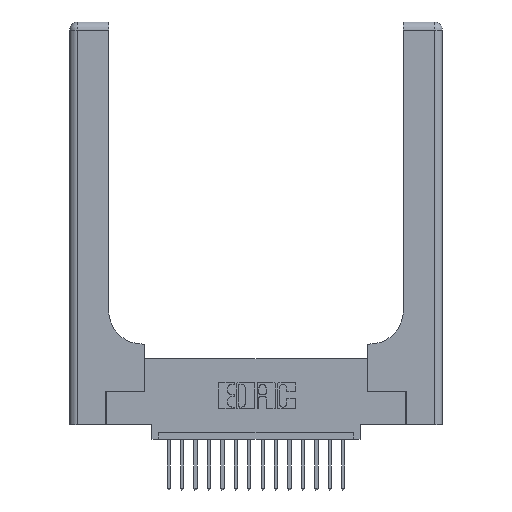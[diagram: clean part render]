
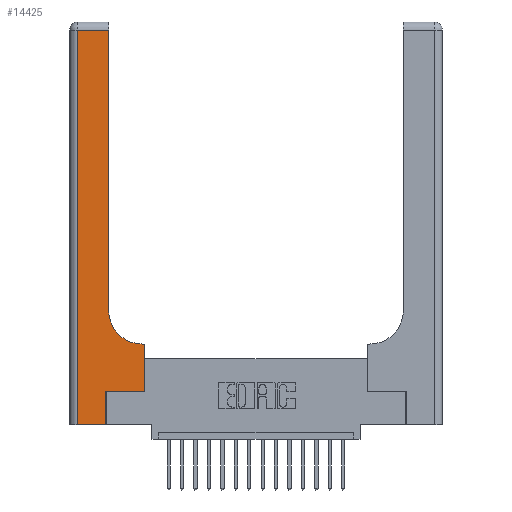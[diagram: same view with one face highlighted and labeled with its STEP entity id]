
A CAD part, top view. The second image highlights one B-rep face of the part: STEP entity #14425.
In plain terms, the highlighted planar face has unit normal (0, 0, 1).
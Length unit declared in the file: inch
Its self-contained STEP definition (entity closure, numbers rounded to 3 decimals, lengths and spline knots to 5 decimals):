
#74 = ORIENTED_EDGE ( 'NONE', *, *, #12690, .T. ) ;
#173 = CARTESIAN_POINT ( 'NONE',  ( 0.269, 0., 0.37 ) ) ;
#455 = CARTESIAN_POINT ( 'NONE',  ( 0.269, 0.25, 0.37 ) ) ;
#500 = EDGE_CURVE ( 'NONE', #16780, #14288, #3269, .T. ) ;
#541 = CARTESIAN_POINT ( 'NONE',  ( 0.5585, 0.25, 0.37 ) ) ;
#1495 = CARTESIAN_POINT ( 'NONE',  ( 0.5585, 0.25, 0.37 ) ) ;
#1512 = CARTESIAN_POINT ( 'NONE',  ( 0.269, 0., 0.37 ) ) ;
#1995 = DIRECTION ( 'NONE',  ( 1., 0., 0. ) ) ;
#2474 = LINE ( 'NONE', #9490, #4388 ) ;
#2658 = EDGE_CURVE ( 'NONE', #5302, #15532, #2474, .T. ) ;
#3269 = LINE ( 'NONE', #1495, #10329 ) ;
#3692 = EDGE_CURVE ( 'NONE', #14288, #13011, #14803, .T. ) ;
#3952 = LINE ( 'NONE', #5649, #6035 ) ;
#4388 = VECTOR ( 'NONE', #17318, 39.37008 ) ;
#4469 = ORIENTED_EDGE ( 'NONE', *, *, #16139, .T. ) ;
#4665 = DIRECTION ( 'NONE',  ( -1., 0., 0. ) ) ;
#4741 = VERTEX_POINT ( 'NONE', #17855 ) ;
#5159 = CARTESIAN_POINT ( 'NONE',  ( 0.2915, 0.6, 0.37 ) ) ;
#5302 = VERTEX_POINT ( 'NONE', #15360 ) ;
#5649 = CARTESIAN_POINT ( 'NONE',  ( 0.2915, 3., 0.37 ) ) ;
#5914 = FACE_OUTER_BOUND ( 'NONE', #9895, .T. ) ;
#5931 = CARTESIAN_POINT ( 'NONE',  ( 0.06, 3., 0.37 ) ) ;
#6035 = VECTOR ( 'NONE', #8735, 39.37008 ) ;
#6331 = VECTOR ( 'NONE', #18338, 39.37008 ) ;
#6656 = ORIENTED_EDGE ( 'NONE', *, *, #500, .T. ) ;
#7239 = EDGE_CURVE ( 'NONE', #13011, #4741, #15145, .T. ) ;
#7361 = DIRECTION ( 'NONE',  ( -1., 0., 0. ) ) ;
#7475 = ORIENTED_EDGE ( 'NONE', *, *, #3692, .T. ) ;
#7903 = CARTESIAN_POINT ( 'NONE',  ( 0.06, 2.94, 0.37 ) ) ;
#7905 = LINE ( 'NONE', #13834, #12405 ) ;
#7948 = CARTESIAN_POINT ( 'NONE',  ( 0.5415, 0.85, 0.37 ) ) ;
#8153 = VECTOR ( 'NONE', #17418, 39.37008 ) ;
#8734 = CARTESIAN_POINT ( 'NONE',  ( 0., 3., 0.37 ) ) ;
#8735 = DIRECTION ( 'NONE',  ( 0., 1., 0. ) ) ;
#8755 = ORIENTED_EDGE ( 'NONE', *, *, #18312, .T. ) ;
#8794 = CARTESIAN_POINT ( 'NONE',  ( 0.5415, 0.6, 0.37 ) ) ;
#9490 = CARTESIAN_POINT ( 'NONE',  ( 0., 0., 0.37 ) ) ;
#9719 = CARTESIAN_POINT ( 'NONE',  ( 0.5585, 0.6, 0.37 ) ) ;
#9895 = EDGE_LOOP ( 'NONE', ( #8755, #11489, #74, #13357, #4469, #10384, #6656, #7475, #17049 ) ) ;
#10180 = VERTEX_POINT ( 'NONE', #7903 ) ;
#10329 = VECTOR ( 'NONE', #18155, 39.37008 ) ;
#10336 = LINE ( 'NONE', #173, #6331 ) ;
#10384 = ORIENTED_EDGE ( 'NONE', *, *, #18777, .T. ) ;
#11489 = ORIENTED_EDGE ( 'NONE', *, *, #11805, .T. ) ;
#11672 = AXIS2_PLACEMENT_3D ( 'NONE', #7948, #12646, #14146 ) ;
#11805 = EDGE_CURVE ( 'NONE', #18182, #10180, #7905, .T. ) ;
#12405 = VECTOR ( 'NONE', #4665, 39.37008 ) ;
#12646 = DIRECTION ( 'NONE',  ( 0., 0., -1. ) ) ;
#12690 = EDGE_CURVE ( 'NONE', #10180, #5302, #13110, .T. ) ;
#13011 = VERTEX_POINT ( 'NONE', #8794 ) ;
#13110 = LINE ( 'NONE', #5931, #14561 ) ;
#13357 = ORIENTED_EDGE ( 'NONE', *, *, #2658, .T. ) ;
#13401 = CARTESIAN_POINT ( 'NONE',  ( 0.269, 0.25, 0.37 ) ) ;
#13470 = CARTESIAN_POINT ( 'NONE',  ( 0.2915, 2.94, 0.37 ) ) ;
#13489 = AXIS2_PLACEMENT_3D ( 'NONE', #8734, #19354, #7361 ) ;
#13834 = CARTESIAN_POINT ( 'NONE',  ( 0., 2.94, 0.37 ) ) ;
#14146 = DIRECTION ( 'NONE',  ( 1., 0., 0. ) ) ;
#14288 = VERTEX_POINT ( 'NONE', #9719 ) ;
#14425 = ADVANCED_FACE ( 'NONE', ( #5914 ), #16582, .F. ) ;
#14561 = VECTOR ( 'NONE', #15182, 39.37008 ) ;
#14803 = LINE ( 'NONE', #5159, #8153 ) ;
#15145 = CIRCLE ( 'NONE', #11672, 0.25 ) ;
#15182 = DIRECTION ( 'NONE',  ( 0., -1., 0. ) ) ;
#15360 = CARTESIAN_POINT ( 'NONE',  ( 0.06, 0., 0.37 ) ) ;
#15532 = VERTEX_POINT ( 'NONE', #1512 ) ;
#16010 = LINE ( 'NONE', #455, #18371 ) ;
#16139 = EDGE_CURVE ( 'NONE', #15532, #17036, #10336, .T. ) ;
#16582 = PLANE ( 'NONE',  #13489 ) ;
#16780 = VERTEX_POINT ( 'NONE', #541 ) ;
#17036 = VERTEX_POINT ( 'NONE', #13401 ) ;
#17049 = ORIENTED_EDGE ( 'NONE', *, *, #7239, .T. ) ;
#17318 = DIRECTION ( 'NONE',  ( 1., 0., 0. ) ) ;
#17418 = DIRECTION ( 'NONE',  ( -1., 0., 0. ) ) ;
#17855 = CARTESIAN_POINT ( 'NONE',  ( 0.2915, 0.85, 0.37 ) ) ;
#18155 = DIRECTION ( 'NONE',  ( 0., 1., 0. ) ) ;
#18182 = VERTEX_POINT ( 'NONE', #13470 ) ;
#18312 = EDGE_CURVE ( 'NONE', #4741, #18182, #3952, .T. ) ;
#18338 = DIRECTION ( 'NONE',  ( 0., 1., 0. ) ) ;
#18371 = VECTOR ( 'NONE', #1995, 39.37008 ) ;
#18777 = EDGE_CURVE ( 'NONE', #17036, #16780, #16010, .T. ) ;
#19354 = DIRECTION ( 'NONE',  ( 0., 0., -1. ) ) ;
